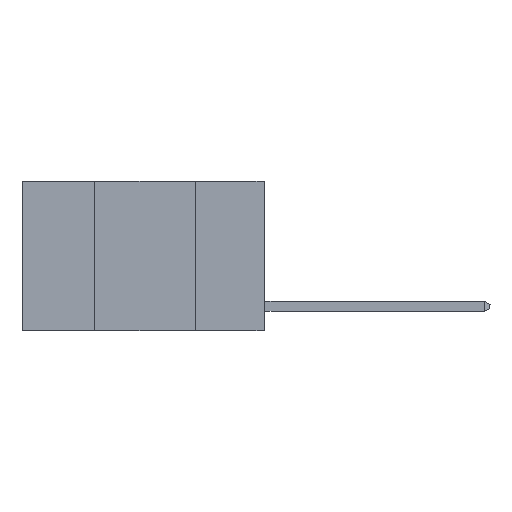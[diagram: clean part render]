
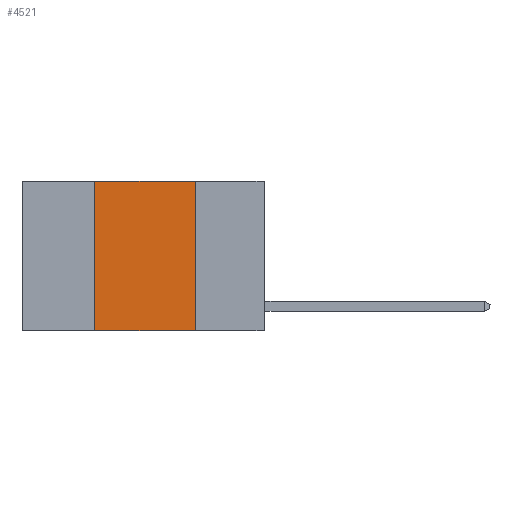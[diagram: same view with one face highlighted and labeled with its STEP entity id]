
A CAD part, left-side view. The second image highlights one B-rep face of the part: STEP entity #4521.
In plain terms, the highlighted planar face has unit normal (-1, 0, 0).
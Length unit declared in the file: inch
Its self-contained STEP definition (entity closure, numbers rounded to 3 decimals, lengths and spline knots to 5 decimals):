
#611 = EDGE_CURVE ( 'NONE', #9377, #19901, #19861, .T. ) ;
#925 = EDGE_LOOP ( 'NONE', ( #6314, #3811, #16581, #7772 ) ) ;
#1197 = DIRECTION ( 'NONE',  ( 0., -1., 0. ) ) ;
#2079 = VECTOR ( 'NONE', #14210, 39.37008 ) ;
#2323 = DIRECTION ( 'NONE',  ( 1., 0., 0. ) ) ;
#3094 = CARTESIAN_POINT ( 'NONE',  ( 0., 0.17, 0. ) ) ;
#3108 = DIRECTION ( 'NONE',  ( 0., -1., 0. ) ) ;
#3179 = CARTESIAN_POINT ( 'NONE',  ( 0., 0.6, 0. ) ) ;
#3811 = ORIENTED_EDGE ( 'NONE', *, *, #8542, .F. ) ;
#4521 = ADVANCED_FACE ( 'NONE', ( #20683 ), #12254, .F. ) ;
#4773 = DIRECTION ( 'NONE',  ( 0., 0., -1. ) ) ;
#5267 = CARTESIAN_POINT ( 'NONE',  ( 0., 0.6, -0.37 ) ) ;
#6314 = ORIENTED_EDGE ( 'NONE', *, *, #13491, .F. ) ;
#6395 = CARTESIAN_POINT ( 'NONE',  ( 0., 0.42, -0.37 ) ) ;
#7213 = VECTOR ( 'NONE', #1197, 39.37008 ) ;
#7772 = ORIENTED_EDGE ( 'NONE', *, *, #611, .T. ) ;
#8542 = EDGE_CURVE ( 'NONE', #12608, #11422, #18757, .T. ) ;
#9169 = CARTESIAN_POINT ( 'NONE',  ( 0., 0.42, 0. ) ) ;
#9377 = VERTEX_POINT ( 'NONE', #6395 ) ;
#10011 = CARTESIAN_POINT ( 'NONE',  ( 0., 0.17, 0. ) ) ;
#10986 = CARTESIAN_POINT ( 'NONE',  ( 0., 0.17, -0.37 ) ) ;
#11422 = VERTEX_POINT ( 'NONE', #10011 ) ;
#12254 = PLANE ( 'NONE',  #13700 ) ;
#12478 = CARTESIAN_POINT ( 'NONE',  ( 0., 0.42, 0. ) ) ;
#12608 = VERTEX_POINT ( 'NONE', #12478 ) ;
#13491 = EDGE_CURVE ( 'NONE', #11422, #19901, #18948, .T. ) ;
#13700 = AXIS2_PLACEMENT_3D ( 'NONE', #17138, #2323, #13927 ) ;
#13927 = DIRECTION ( 'NONE',  ( 0., 0., -1. ) ) ;
#14210 = DIRECTION ( 'NONE',  ( 0., 0., 1. ) ) ;
#14606 = VECTOR ( 'NONE', #4773, 39.37008 ) ;
#14926 = VECTOR ( 'NONE', #3108, 39.37008 ) ;
#16581 = ORIENTED_EDGE ( 'NONE', *, *, #19190, .F. ) ;
#17138 = CARTESIAN_POINT ( 'NONE',  ( 0., 0.6, 0. ) ) ;
#18757 = LINE ( 'NONE', #3179, #14926 ) ;
#18948 = LINE ( 'NONE', #3094, #14606 ) ;
#19190 = EDGE_CURVE ( 'NONE', #9377, #12608, #20639, .T. ) ;
#19861 = LINE ( 'NONE', #5267, #7213 ) ;
#19901 = VERTEX_POINT ( 'NONE', #10986 ) ;
#20639 = LINE ( 'NONE', #9169, #2079 ) ;
#20683 = FACE_OUTER_BOUND ( 'NONE', #925, .T. ) ;
